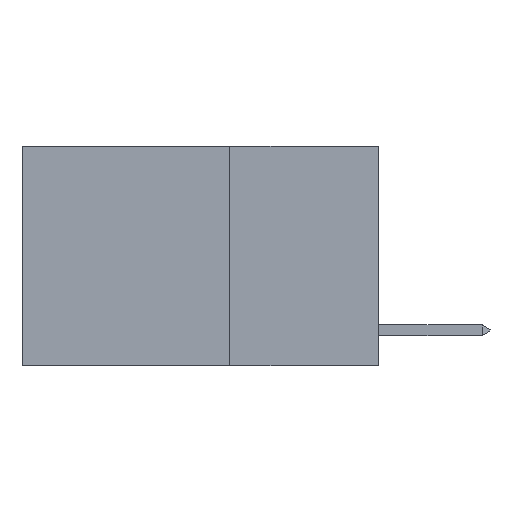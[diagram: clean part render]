
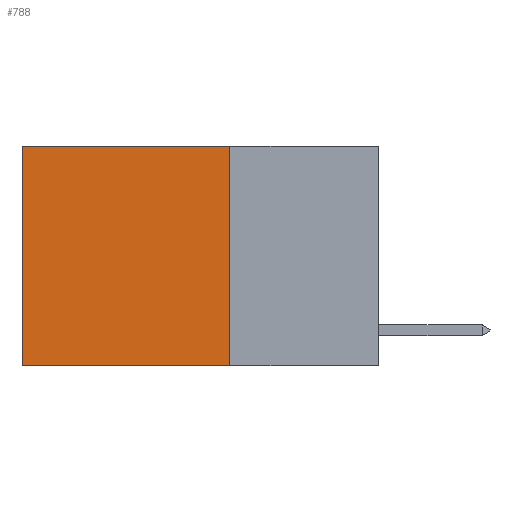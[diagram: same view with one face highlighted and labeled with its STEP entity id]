
A CAD part, left-side view. The second image highlights one B-rep face of the part: STEP entity #788.
In plain terms, the highlighted planar face has unit normal (-1, 0, 0).
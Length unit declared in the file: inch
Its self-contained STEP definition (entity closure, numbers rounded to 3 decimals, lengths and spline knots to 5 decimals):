
#32 = CARTESIAN_POINT ( 'NONE',  ( 0.2625, 0.25, 0. ) ) ;
#323 = ORIENTED_EDGE ( 'NONE', *, *, #11127, .F. ) ;
#649 = VERTEX_POINT ( 'NONE', #4474 ) ;
#788 = ADVANCED_FACE ( 'NONE', ( #17074 ), #3137, .F. ) ;
#1159 = EDGE_CURVE ( 'NONE', #649, #18055, #18398, .T. ) ;
#1809 = CARTESIAN_POINT ( 'NONE',  ( 0.2625, 0.6, 0. ) ) ;
#2210 = DIRECTION ( 'NONE',  ( 0., 1., 0. ) ) ;
#2588 = ORIENTED_EDGE ( 'NONE', *, *, #19485, .T. ) ;
#3071 = DIRECTION ( 'NONE',  ( 0., 0., -1. ) ) ;
#3118 = DIRECTION ( 'NONE',  ( 1., 0., 0. ) ) ;
#3137 = PLANE ( 'NONE',  #11921 ) ;
#3287 = CARTESIAN_POINT ( 'NONE',  ( 0.2625, 0.25, 0. ) ) ;
#3739 = CARTESIAN_POINT ( 'NONE',  ( 0.2625, 0.25, 0. ) ) ;
#4474 = CARTESIAN_POINT ( 'NONE',  ( 0.2625, 0.6, 0. ) ) ;
#6265 = ORIENTED_EDGE ( 'NONE', *, *, #13800, .F. ) ;
#6495 = VERTEX_POINT ( 'NONE', #3739 ) ;
#6633 = VECTOR ( 'NONE', #7128, 39.37008 ) ;
#7128 = DIRECTION ( 'NONE',  ( 0., 0., -1. ) ) ;
#7502 = VECTOR ( 'NONE', #2210, 39.37008 ) ;
#9107 = VECTOR ( 'NONE', #16879, 39.37008 ) ;
#10506 = ORIENTED_EDGE ( 'NONE', *, *, #1159, .T. ) ;
#10630 = LINE ( 'NONE', #32, #18605 ) ;
#10777 = CARTESIAN_POINT ( 'NONE',  ( 0.2625, 0.25, 0. ) ) ;
#11127 = EDGE_CURVE ( 'NONE', #12658, #18055, #15807, .T. ) ;
#11921 = AXIS2_PLACEMENT_3D ( 'NONE', #3287, #3118, #3071 ) ;
#12658 = VERTEX_POINT ( 'NONE', #17760 ) ;
#13295 = LINE ( 'NONE', #10777, #9107 ) ;
#13800 = EDGE_CURVE ( 'NONE', #6495, #12658, #10630, .T. ) ;
#14429 = DIRECTION ( 'NONE',  ( 0., 0., -1. ) ) ;
#15807 = LINE ( 'NONE', #17816, #7502 ) ;
#16879 = DIRECTION ( 'NONE',  ( 0., 1., 0. ) ) ;
#17074 = FACE_OUTER_BOUND ( 'NONE', #17352, .T. ) ;
#17352 = EDGE_LOOP ( 'NONE', ( #10506, #323, #6265, #2588 ) ) ;
#17617 = CARTESIAN_POINT ( 'NONE',  ( 0.2625, 0.6, -0.37 ) ) ;
#17760 = CARTESIAN_POINT ( 'NONE',  ( 0.2625, 0.25, -0.37 ) ) ;
#17816 = CARTESIAN_POINT ( 'NONE',  ( 0.2625, 0.25, -0.37 ) ) ;
#18055 = VERTEX_POINT ( 'NONE', #17617 ) ;
#18398 = LINE ( 'NONE', #1809, #6633 ) ;
#18605 = VECTOR ( 'NONE', #14429, 39.37008 ) ;
#19485 = EDGE_CURVE ( 'NONE', #6495, #649, #13295, .T. ) ;
